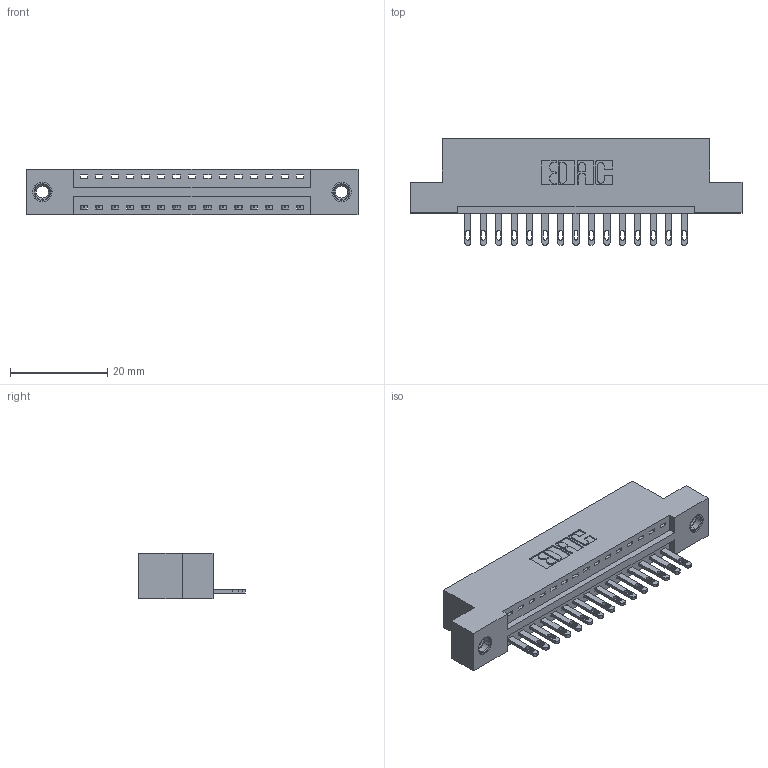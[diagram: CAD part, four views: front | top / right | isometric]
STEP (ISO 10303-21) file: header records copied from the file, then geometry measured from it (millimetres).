
FILE_DESCRIPTION (( 'STEP AP203' ), '1' );
FILE_NAME ('896-015-500-107.STEP', '2021-07-27T15:26:11', ( '' ), ( '' ), 'SwSTEP 2.0', 'SolidWorks 2020', '' );
FILE_SCHEMA (( 'CONFIG_CONTROL_DESIGN' ));
Length unit declared in the file: inch
Products named in the file (4): 345-292-001_345-293-100; 345-250-001_345-250-005-103; 846 Part_Flush Mounting Lugs - 0.156 Dia-TI; 896-015-500-107
Assembly tree (18 placements, depth 2):
  896-015-500-107
    846 Part_Flush Mounting Lugs - 0.156 Dia-TI
    345-292-001_345-293-100  x15
    345-250-001_345-250-005-103  x2
Bounding box: 68.2 x 21.84 x 9.4 mm (x, y, z)
Volume: 6337.9 mm3; surface area: 7699.8 mm2
Topology: 18 solids, 18 shells, 992 faces, 2985 edges, 1982 vertices
Faces by surface type: plane 618, cylinder 358, cone 12, torus 4
Entity records: 14060 total; most frequent: CARTESIAN_POINT 2400, ORIENTED_EDGE 2342, DIRECTION 2179, EDGE_CURVE 1171, VECTOR 955, LINE 955, VERTEX_POINT 776, AXIS2_PLACEMENT_3D 612
